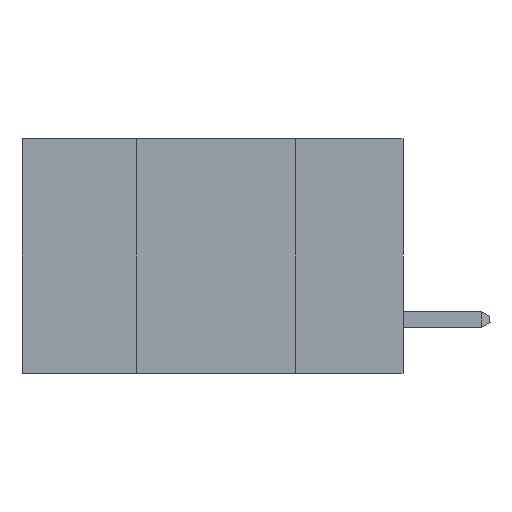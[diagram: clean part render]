
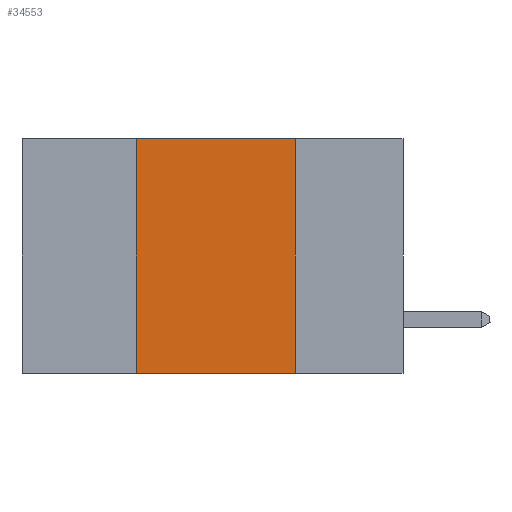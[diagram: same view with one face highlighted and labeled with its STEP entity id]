
A CAD part, left-side view. The second image highlights one B-rep face of the part: STEP entity #34553.
In plain terms, the highlighted planar face has unit normal (-1, 0, 0).
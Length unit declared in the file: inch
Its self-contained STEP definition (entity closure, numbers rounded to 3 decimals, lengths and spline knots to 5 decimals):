
#424 = FACE_OUTER_BOUND ( 'NONE', #3738, .T. ) ;
#759 = CARTESIAN_POINT ( 'NONE',  ( 0., 0.42, 0. ) ) ;
#1466 = LINE ( 'NONE', #45472, #10807 ) ;
#3738 = EDGE_LOOP ( 'NONE', ( #19999, #47568, #31127, #35143 ) ) ;
#7331 = EDGE_CURVE ( 'NONE', #33181, #35896, #1466, .T. ) ;
#10807 = VECTOR ( 'NONE', #30147, 39.37008 ) ;
#11775 = DIRECTION ( 'NONE',  ( 1., 0., 0. ) ) ;
#11961 = CARTESIAN_POINT ( 'NONE',  ( 0., 0.6, 0. ) ) ;
#12342 = CARTESIAN_POINT ( 'NONE',  ( 0., 0.17, -0.37 ) ) ;
#12890 = DIRECTION ( 'NONE',  ( 0., 0., 1. ) ) ;
#15284 = DIRECTION ( 'NONE',  ( 0., 0., -1. ) ) ;
#15979 = DIRECTION ( 'NONE',  ( 0., -1., 0. ) ) ;
#19705 = LINE ( 'NONE', #32460, #38956 ) ;
#19999 = ORIENTED_EDGE ( 'NONE', *, *, #34027, .F. ) ;
#22527 = VERTEX_POINT ( 'NONE', #43457 ) ;
#25341 = AXIS2_PLACEMENT_3D ( 'NONE', #43548, #11775, #15284 ) ;
#28807 = EDGE_CURVE ( 'NONE', #33181, #35341, #19705, .T. ) ;
#30147 = DIRECTION ( 'NONE',  ( 0., -1., 0. ) ) ;
#30502 = VECTOR ( 'NONE', #15979, 39.37008 ) ;
#31127 = ORIENTED_EDGE ( 'NONE', *, *, #28807, .F. ) ;
#31357 = VECTOR ( 'NONE', #36468, 39.37008 ) ;
#32460 = CARTESIAN_POINT ( 'NONE',  ( 0., 0.42, 0. ) ) ;
#32538 = EDGE_CURVE ( 'NONE', #35341, #22527, #46682, .T. ) ;
#32790 = CARTESIAN_POINT ( 'NONE',  ( 0., 0.17, 0. ) ) ;
#33181 = VERTEX_POINT ( 'NONE', #44015 ) ;
#34027 = EDGE_CURVE ( 'NONE', #22527, #35896, #41954, .T. ) ;
#34553 = ADVANCED_FACE ( 'NONE', ( #424 ), #39073, .F. ) ;
#35143 = ORIENTED_EDGE ( 'NONE', *, *, #7331, .T. ) ;
#35341 = VERTEX_POINT ( 'NONE', #759 ) ;
#35896 = VERTEX_POINT ( 'NONE', #12342 ) ;
#36468 = DIRECTION ( 'NONE',  ( 0., 0., -1. ) ) ;
#38956 = VECTOR ( 'NONE', #12890, 39.37008 ) ;
#39073 = PLANE ( 'NONE',  #25341 ) ;
#41954 = LINE ( 'NONE', #32790, #31357 ) ;
#43457 = CARTESIAN_POINT ( 'NONE',  ( 0., 0.17, 0. ) ) ;
#43548 = CARTESIAN_POINT ( 'NONE',  ( 0., 0.6, 0. ) ) ;
#44015 = CARTESIAN_POINT ( 'NONE',  ( 0., 0.42, -0.37 ) ) ;
#45472 = CARTESIAN_POINT ( 'NONE',  ( 0., 0.6, -0.37 ) ) ;
#46682 = LINE ( 'NONE', #11961, #30502 ) ;
#47568 = ORIENTED_EDGE ( 'NONE', *, *, #32538, .F. ) ;
